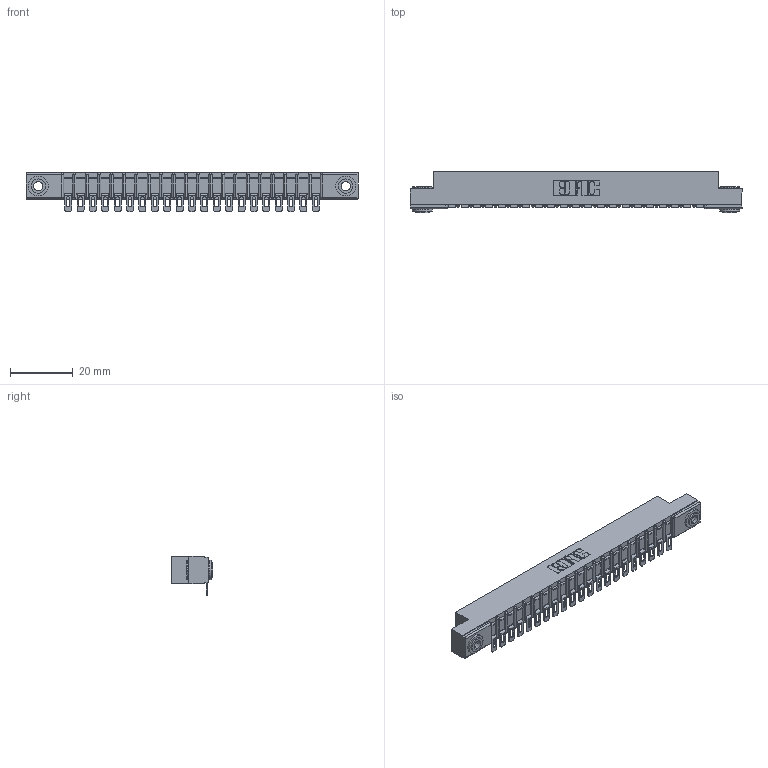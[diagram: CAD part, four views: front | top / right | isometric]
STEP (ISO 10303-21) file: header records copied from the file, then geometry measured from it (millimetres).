
FILE_DESCRIPTION (( 'STEP AP203' ), '1' );
FILE_NAME ('357-021-554-103.STEP', '2019-09-16T22:54:22', ( '' ), ( '' ), 'SwSTEP 2.0', 'SolidWorks 2016', '' );
FILE_SCHEMA (( 'CONFIG_CONTROL_DESIGN' ));
Length unit declared in the file: inch
Products named in the file (4): 345-250-002_345-250-002-102; 357-021-554-103; 307 Part_.156 Dia Mounting Holes; 307-290-002_554
Assembly tree (24 placements, depth 2):
  357-021-554-103
    307 Part_.156 Dia Mounting Holes
    307-290-002_554  x21
    345-250-002_345-250-002-102  x2
Bounding box: 106.22 x 13.36 x 12.52 mm (x, y, z)
Volume: 7021 mm3; surface area: 13044.7 mm2
Topology: 24 solids, 24 shells, 1893 faces, 5748 edges, 3768 vertices
Faces by surface type: plane 1060, cylinder 781, sphere 44, cone 8
Entity records: 22622 total; most frequent: CARTESIAN_POINT 3791, ORIENTED_EDGE 3772, DIRECTION 3714, EDGE_CURVE 1886, LINE 1420, VECTOR 1420, VERTEX_POINT 1224, AXIS2_PLACEMENT_3D 1147
